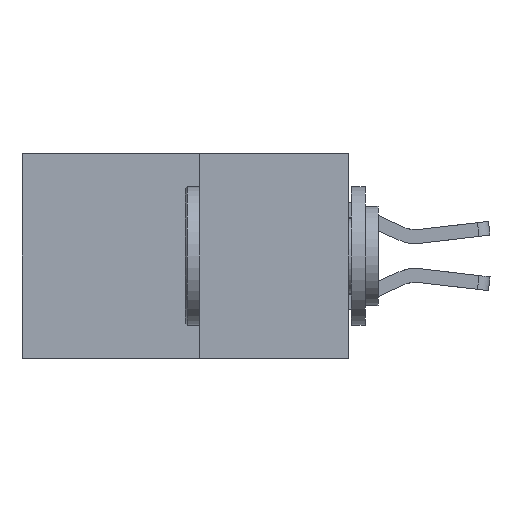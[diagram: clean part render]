
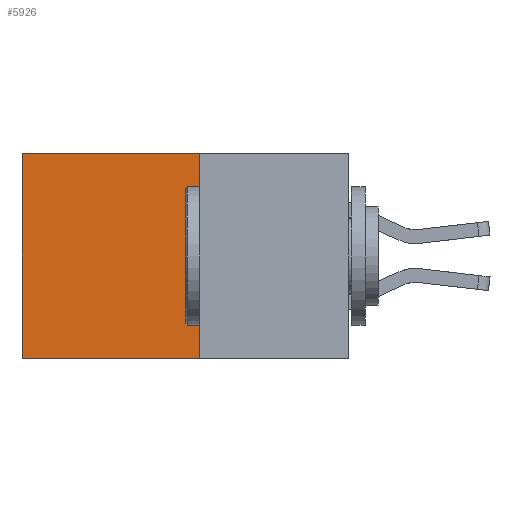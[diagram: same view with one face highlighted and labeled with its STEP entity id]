
A CAD part, left-side view. The second image highlights one B-rep face of the part: STEP entity #5926.
In plain terms, the highlighted planar face has unit normal (-1, 0, 0).
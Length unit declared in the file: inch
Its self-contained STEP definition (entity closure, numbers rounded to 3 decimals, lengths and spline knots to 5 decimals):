
#574 = CARTESIAN_POINT ( 'NONE',  ( 0.277, 0.27, -0.37 ) ) ;
#864 = ORIENTED_EDGE ( 'NONE', *, *, #4587, .T. ) ;
#997 = DIRECTION ( 'NONE',  ( 0., 1., 0. ) ) ;
#1030 = CARTESIAN_POINT ( 'NONE',  ( 0.277, 0.27, -0.37 ) ) ;
#1983 = AXIS2_PLACEMENT_3D ( 'NONE', #8704, #8486, #8471 ) ;
#2221 = VECTOR ( 'NONE', #7047, 39.37008 ) ;
#2301 = CARTESIAN_POINT ( 'NONE',  ( 0.277, 0.59, -0.37 ) ) ;
#2323 = ORIENTED_EDGE ( 'NONE', *, *, #7512, .T. ) ;
#2374 = ORIENTED_EDGE ( 'NONE', *, *, #7857, .F. ) ;
#2416 = ORIENTED_EDGE ( 'NONE', *, *, #11025, .F. ) ;
#2752 = FACE_OUTER_BOUND ( 'NONE', #4388, .T. ) ;
#3118 = LINE ( 'NONE', #4717, #5190 ) ;
#3276 = VERTEX_POINT ( 'NONE', #2301 ) ;
#3444 = CARTESIAN_POINT ( 'NONE',  ( 0.277, 0.59, 0. ) ) ;
#3522 = CARTESIAN_POINT ( 'NONE',  ( 0.277, 0.27, 0. ) ) ;
#3877 = DIRECTION ( 'NONE',  ( 0., 1., 0. ) ) ;
#3943 = VECTOR ( 'NONE', #997, 39.37008 ) ;
#4388 = EDGE_LOOP ( 'NONE', ( #2323, #2374, #2416, #864 ) ) ;
#4401 = LINE ( 'NONE', #5339, #6408 ) ;
#4541 = LINE ( 'NONE', #9712, #2221 ) ;
#4587 = EDGE_CURVE ( 'NONE', #9798, #6242, #4401, .T. ) ;
#4672 = DIRECTION ( 'NONE',  ( 0., 0., -1. ) ) ;
#4717 = CARTESIAN_POINT ( 'NONE',  ( 0.277, 0.59, -0.37 ) ) ;
#5099 = VERTEX_POINT ( 'NONE', #574 ) ;
#5190 = VECTOR ( 'NONE', #4672, 39.37008 ) ;
#5339 = CARTESIAN_POINT ( 'NONE',  ( 0.277, 0.27, 0. ) ) ;
#5926 = ADVANCED_FACE ( 'NONE', ( #2752 ), #8629, .F. ) ;
#6242 = VERTEX_POINT ( 'NONE', #3444 ) ;
#6408 = VECTOR ( 'NONE', #3877, 39.37008 ) ;
#7047 = DIRECTION ( 'NONE',  ( 0., 0., -1. ) ) ;
#7512 = EDGE_CURVE ( 'NONE', #6242, #3276, #3118, .T. ) ;
#7857 = EDGE_CURVE ( 'NONE', #5099, #3276, #8608, .T. ) ;
#8471 = DIRECTION ( 'NONE',  ( 0., 0., -1. ) ) ;
#8486 = DIRECTION ( 'NONE',  ( 1., 0., 0. ) ) ;
#8608 = LINE ( 'NONE', #1030, #3943 ) ;
#8629 = PLANE ( 'NONE',  #1983 ) ;
#8704 = CARTESIAN_POINT ( 'NONE',  ( 0.277, 0.27, -0.37 ) ) ;
#9712 = CARTESIAN_POINT ( 'NONE',  ( 0.277, 0.27, -0.37 ) ) ;
#9798 = VERTEX_POINT ( 'NONE', #3522 ) ;
#11025 = EDGE_CURVE ( 'NONE', #9798, #5099, #4541, .T. ) ;
